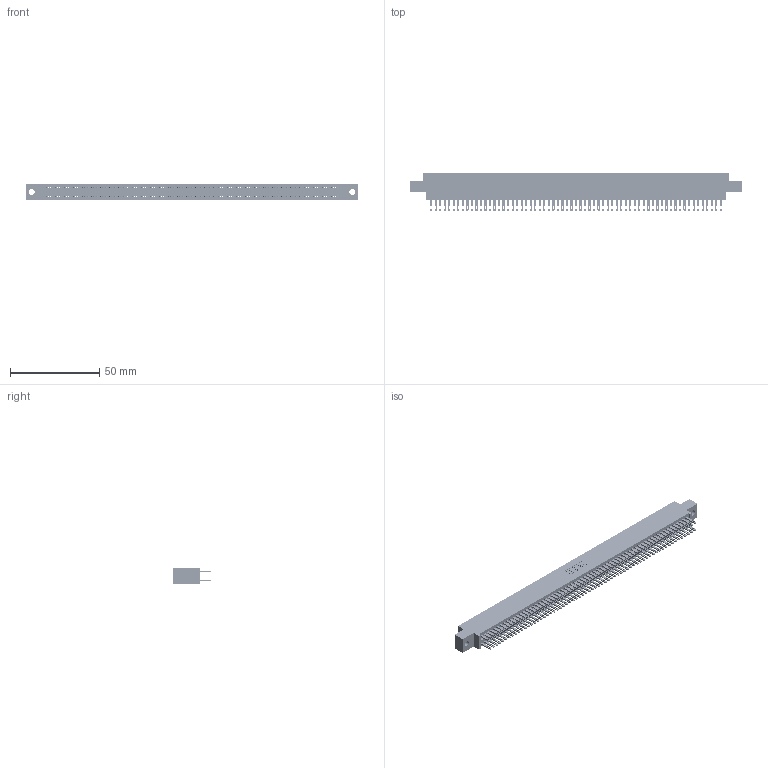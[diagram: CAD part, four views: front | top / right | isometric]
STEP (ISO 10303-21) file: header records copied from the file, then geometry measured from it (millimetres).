
FILE_DESCRIPTION (( 'STEP AP203' ), '1' );
FILE_NAME ('895-130-500-802.STEP', '2020-10-13T17:10:40', ( '' ), ( '' ), 'SwSTEP 2.0', 'SolidWorks 2020', '' );
FILE_SCHEMA (( 'CONFIG_CONTROL_DESIGN' ));
Length unit declared in the file: inch
Products named in the file (3): 345-292-001_345-293-100; 895-130-500-802; 845 Part_0.170 Offset - 0.128 Dia
Assembly tree (131 placements, depth 2):
  895-130-500-802
    845 Part_0.170 Offset - 0.128 Dia
    345-292-001_345-293-100  x130
Bounding box: 186.31 x 21.51 x 9.4 mm (x, y, z)
Volume: 18558.9 mm3; surface area: 29075.3 mm2
Topology: 131 solids, 131 shells, 6110 faces, 18683 edges, 12454 vertices
Faces by surface type: plane 3594, cylinder 2516
Entity records: 47969 total; most frequent: CARTESIAN_POINT 8020, ORIENTED_EDGE 7954, DIRECTION 7045, EDGE_CURVE 3977, LINE 3581, VECTOR 3581, VERTEX_POINT 2650, AXIS2_PLACEMENT_3D 1732
